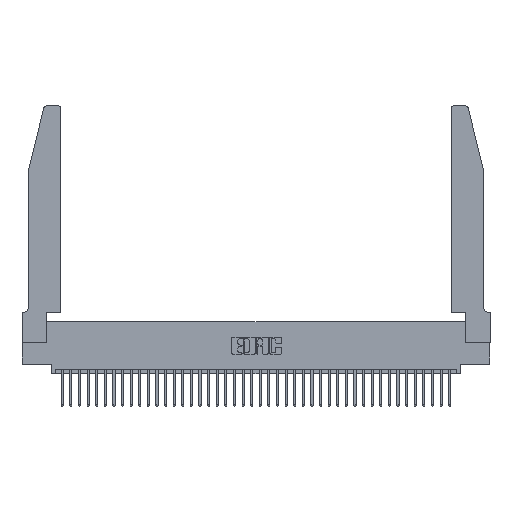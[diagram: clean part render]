
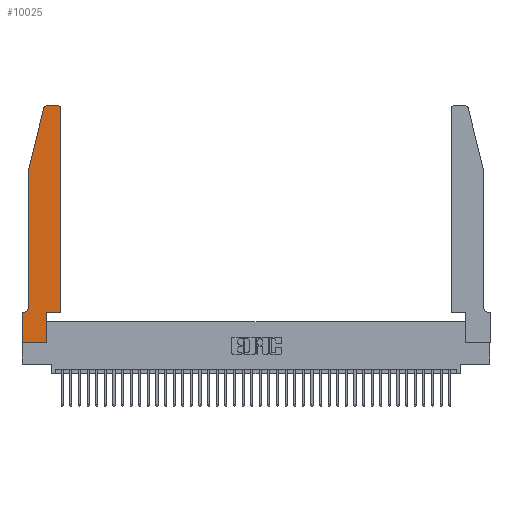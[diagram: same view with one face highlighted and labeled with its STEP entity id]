
A CAD part, top view. The second image highlights one B-rep face of the part: STEP entity #10025.
In plain terms, the highlighted planar face has unit normal (0, 0, 1).
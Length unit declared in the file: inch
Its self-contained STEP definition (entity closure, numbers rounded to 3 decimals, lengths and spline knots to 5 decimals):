
#497 = VECTOR ( 'NONE', #2498, 39.37008 ) ;
#870 = CIRCLE ( 'NONE', #1994, 0.07 ) ;
#889 = ORIENTED_EDGE ( 'NONE', *, *, #18268, .T. ) ;
#1182 = VERTEX_POINT ( 'NONE', #12669 ) ;
#1297 = CARTESIAN_POINT ( 'NONE',  ( 0.25487, 2.72718, 0.37 ) ) ;
#1478 = VECTOR ( 'NONE', #25336, 39.37008 ) ;
#1632 = VERTEX_POINT ( 'NONE', #1297 ) ;
#1994 = AXIS2_PLACEMENT_3D ( 'NONE', #18825, #24239, #3602 ) ;
#2106 = CARTESIAN_POINT ( 'NONE',  ( 0.4505, 0.35, 0.37 ) ) ;
#2498 = DIRECTION ( 'NONE',  ( 1., 0., 0. ) ) ;
#2580 = CARTESIAN_POINT ( 'NONE',  ( 0.4505, 2.72, 0.37 ) ) ;
#3012 = VERTEX_POINT ( 'NONE', #2580 ) ;
#3232 = CARTESIAN_POINT ( 'NONE',  ( 0.284, 2.75, 0.37 ) ) ;
#3581 = LINE ( 'NONE', #16673, #8951 ) ;
#3602 = DIRECTION ( 'NONE',  ( -1., 0., 0. ) ) ;
#3929 = LINE ( 'NONE', #2106, #497 ) ;
#4255 = FACE_OUTER_BOUND ( 'NONE', #40120, .T. ) ;
#4391 = VERTEX_POINT ( 'NONE', #14918 ) ;
#4629 = DIRECTION ( 'NONE',  ( -1., 0., 0. ) ) ;
#4735 = AXIS2_PLACEMENT_3D ( 'NONE', #12414, #13070, #19803 ) ;
#6829 = CARTESIAN_POINT ( 'NONE',  ( 0.2865, 0., 0.37 ) ) ;
#7659 = VECTOR ( 'NONE', #16834, 39.37008 ) ;
#8167 = EDGE_CURVE ( 'NONE', #3012, #40214, #33768, .T. ) ;
#8582 = DIRECTION ( 'NONE',  ( 0., 1., 0. ) ) ;
#8793 = CARTESIAN_POINT ( 'NONE',  ( 0.0055, 0.35, 0.37 ) ) ;
#8838 = CARTESIAN_POINT ( 'NONE',  ( 0.284, 2.72, 0.37 ) ) ;
#8951 = VECTOR ( 'NONE', #4629, 39.37008 ) ;
#9004 = ORIENTED_EDGE ( 'NONE', *, *, #27176, .T. ) ;
#9091 = ORIENTED_EDGE ( 'NONE', *, *, #8167, .T. ) ;
#9470 = VECTOR ( 'NONE', #20917, 39.37008 ) ;
#10025 = ADVANCED_FACE ( 'NONE', ( #4255 ), #14411, .T. ) ;
#10382 = CIRCLE ( 'NONE', #19714, 0.03 ) ;
#10775 = CARTESIAN_POINT ( 'NONE',  ( 0.0755, 2., 0.37 ) ) ;
#11467 = CARTESIAN_POINT ( 'NONE',  ( 0.2865, 0.35, 0.37 ) ) ;
#11613 = EDGE_CURVE ( 'NONE', #30761, #4391, #34467, .T. ) ;
#12318 = EDGE_CURVE ( 'NONE', #18306, #21760, #36867, .T. ) ;
#12414 = CARTESIAN_POINT ( 'NONE',  ( 0.4205, 2.72, 0.37 ) ) ;
#12669 = CARTESIAN_POINT ( 'NONE',  ( 0.4505, 0.35, 0.37 ) ) ;
#12811 = VECTOR ( 'NONE', #13087, 39.37008 ) ;
#13070 = DIRECTION ( 'NONE',  ( 0., 0., 1. ) ) ;
#13087 = DIRECTION ( 'NONE',  ( 0., -1., 0. ) ) ;
#13723 = DIRECTION ( 'NONE',  ( -0.239, -0.971, 0. ) ) ;
#13838 = EDGE_CURVE ( 'NONE', #40214, #20939, #16128, .T. ) ;
#14411 = PLANE ( 'NONE',  #22818 ) ;
#14654 = EDGE_CURVE ( 'NONE', #4391, #21542, #870, .T. ) ;
#14712 = DIRECTION ( 'NONE',  ( 1., 0., 0. ) ) ;
#14871 = CARTESIAN_POINT ( 'NONE',  ( 0., 0.35, 0.37 ) ) ;
#14918 = CARTESIAN_POINT ( 'NONE',  ( 0.0755, 0.42, 0.37 ) ) ;
#15427 = VECTOR ( 'NONE', #22427, 39.37008 ) ;
#15614 = ORIENTED_EDGE ( 'NONE', *, *, #31844, .T. ) ;
#16128 = LINE ( 'NONE', #37629, #1478 ) ;
#16673 = CARTESIAN_POINT ( 'NONE',  ( 0.0755, 0.35, 0.37 ) ) ;
#16834 = DIRECTION ( 'NONE',  ( 0., 1., 0. ) ) ;
#17872 = CARTESIAN_POINT ( 'NONE',  ( 0., 0.35, 0.37 ) ) ;
#18268 = EDGE_CURVE ( 'NONE', #21542, #18306, #3581, .T. ) ;
#18306 = VERTEX_POINT ( 'NONE', #14871 ) ;
#18634 = ORIENTED_EDGE ( 'NONE', *, *, #14654, .T. ) ;
#18825 = CARTESIAN_POINT ( 'NONE',  ( 0.0055, 0.42, 0.37 ) ) ;
#19303 = VECTOR ( 'NONE', #13723, 39.37008 ) ;
#19349 = EDGE_CURVE ( 'NONE', #20357, #1182, #3929, .T. ) ;
#19714 = AXIS2_PLACEMENT_3D ( 'NONE', #8838, #33642, #14712 ) ;
#19803 = DIRECTION ( 'NONE',  ( 1., 0., 0. ) ) ;
#20357 = VERTEX_POINT ( 'NONE', #24223 ) ;
#20917 = DIRECTION ( 'NONE',  ( 0., -1., 0. ) ) ;
#20939 = VERTEX_POINT ( 'NONE', #3232 ) ;
#21542 = VERTEX_POINT ( 'NONE', #8793 ) ;
#21720 = CARTESIAN_POINT ( 'NONE',  ( 0.0755, 2., 0.37 ) ) ;
#21760 = VERTEX_POINT ( 'NONE', #27952 ) ;
#21869 = VERTEX_POINT ( 'NONE', #6829 ) ;
#22300 = LINE ( 'NONE', #31616, #15427 ) ;
#22427 = DIRECTION ( 'NONE',  ( 1., 0., 0. ) ) ;
#22818 = AXIS2_PLACEMENT_3D ( 'NONE', #17872, #36744, #40008 ) ;
#23321 = ORIENTED_EDGE ( 'NONE', *, *, #33857, .T. ) ;
#24223 = CARTESIAN_POINT ( 'NONE',  ( 0.2865, 0.35, 0.37 ) ) ;
#24239 = DIRECTION ( 'NONE',  ( 0., 0., -1. ) ) ;
#24315 = EDGE_CURVE ( 'NONE', #21760, #21869, #22300, .T. ) ;
#25336 = DIRECTION ( 'NONE',  ( -1., 0., 0. ) ) ;
#25525 = CARTESIAN_POINT ( 'NONE',  ( 0.4205, 2.75, 0.37 ) ) ;
#26293 = VECTOR ( 'NONE', #8582, 39.37008 ) ;
#26557 = ORIENTED_EDGE ( 'NONE', *, *, #24315, .T. ) ;
#26964 = ORIENTED_EDGE ( 'NONE', *, *, #13838, .T. ) ;
#27176 = EDGE_CURVE ( 'NONE', #20939, #1632, #10382, .T. ) ;
#27952 = CARTESIAN_POINT ( 'NONE',  ( 0., 0., 0.37 ) ) ;
#29185 = CARTESIAN_POINT ( 'NONE',  ( 0.0755, 2., 0.37 ) ) ;
#29800 = EDGE_CURVE ( 'NONE', #1182, #3012, #38051, .T. ) ;
#30761 = VERTEX_POINT ( 'NONE', #21720 ) ;
#31616 = CARTESIAN_POINT ( 'NONE',  ( 0., 0., 0.37 ) ) ;
#31844 = EDGE_CURVE ( 'NONE', #21869, #20357, #36640, .T. ) ;
#32298 = CARTESIAN_POINT ( 'NONE',  ( 0.4505, 0.35, 0.37 ) ) ;
#32418 = CARTESIAN_POINT ( 'NONE',  ( 0., 0., 0.37 ) ) ;
#33032 = LINE ( 'NONE', #29185, #19303 ) ;
#33642 = DIRECTION ( 'NONE',  ( 0., 0., 1. ) ) ;
#33768 = CIRCLE ( 'NONE', #4735, 0.03 ) ;
#33857 = EDGE_CURVE ( 'NONE', #1632, #30761, #33032, .T. ) ;
#33862 = ORIENTED_EDGE ( 'NONE', *, *, #19349, .T. ) ;
#34467 = LINE ( 'NONE', #10775, #9470 ) ;
#36640 = LINE ( 'NONE', #11467, #26293 ) ;
#36744 = DIRECTION ( 'NONE',  ( 0., 0., 1. ) ) ;
#36867 = LINE ( 'NONE', #32418, #12811 ) ;
#37391 = ORIENTED_EDGE ( 'NONE', *, *, #29800, .T. ) ;
#37629 = CARTESIAN_POINT ( 'NONE',  ( 0.2605, 2.75, 0.37 ) ) ;
#38051 = LINE ( 'NONE', #32298, #7659 ) ;
#39587 = ORIENTED_EDGE ( 'NONE', *, *, #12318, .T. ) ;
#39731 = ORIENTED_EDGE ( 'NONE', *, *, #11613, .T. ) ;
#40008 = DIRECTION ( 'NONE',  ( 1., 0., 0. ) ) ;
#40120 = EDGE_LOOP ( 'NONE', ( #26964, #9004, #23321, #39731, #18634, #889, #39587, #26557, #15614, #33862, #37391, #9091 ) ) ;
#40214 = VERTEX_POINT ( 'NONE', #25525 ) ;
